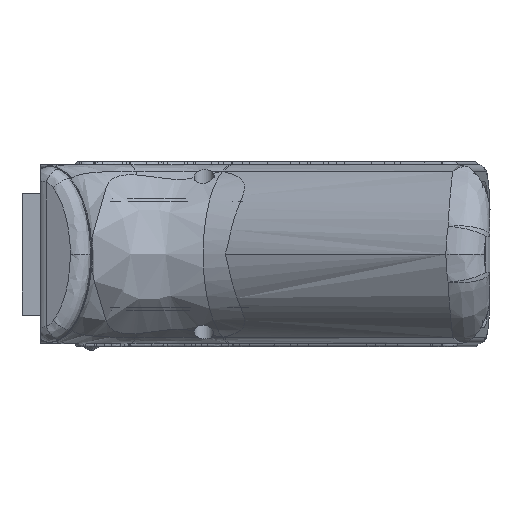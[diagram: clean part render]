
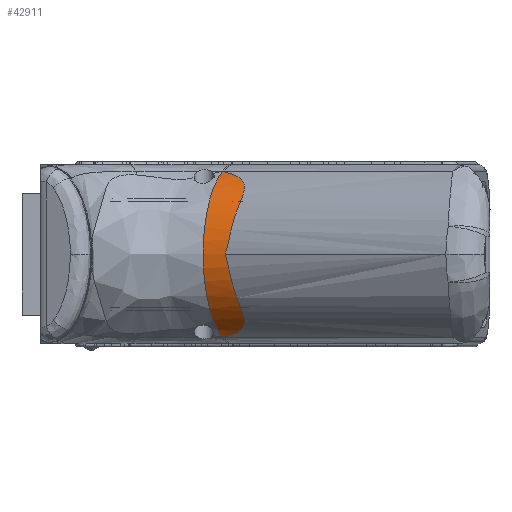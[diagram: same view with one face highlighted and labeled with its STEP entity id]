
A CAD part, left-side view. The second image highlights one B-rep face of the part: STEP entity #42911.
In plain terms, the highlighted free-form (B-spline) face has degree [2, 1] with [5, 2] control points.
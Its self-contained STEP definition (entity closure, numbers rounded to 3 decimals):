
#154=(
BOUNDED_SURFACE()
B_SPLINE_SURFACE(2,1,((#91286,#91287),(#91288,#91289),(#91290,#91291),(#91292,
#91293),(#91294,#91295)),.UNSPECIFIED.,.F.,.F.,.F.)
B_SPLINE_SURFACE_WITH_KNOTS((3,2,3),(2,2),(-2.705,-1.571,
-0.437),(0.,1.202),.UNSPECIFIED.)
GEOMETRIC_REPRESENTATION_ITEM()
RATIONAL_B_SPLINE_SURFACE(((1.,1.),(0.843,0.843),
(1.,1.),(0.843,0.843),(1.,1.)))
REPRESENTATION_ITEM('')
SURFACE()
);
#941=CIRCLE('',#45592,14.75);
#942=CIRCLE('',#45593,14.75);
#943=CIRCLE('',#45594,14.75);
#1328=B_SPLINE_CURVE_WITH_KNOTS('',3,(#60551,#60552,#60553,#60554,#60555,
#60556,#60557,#60558,#60559,#60560,#60561,#60562,#60563,#60564,#60565,#60566,
#60567,#60568,#60569,#60570,#60571,#60572,#60573,#60574,#60575,#60576,#60577,
#60578,#60579,#60580,#60581,#60582,#60583,#60584),.UNSPECIFIED.,.F.,.F.,
(4,2,2,2,2,2,2,2,2,2,2,2,2,2,2,2,4),(-1.682,-1.681,
-1.679,-1.676,-1.669,-1.656,
-1.628,-1.57,-1.446,-1.192,
-0.918,-0.77,-0.689,-0.595,
-0.408,-0.204,0.),.UNSPECIFIED.);
#1333=B_SPLINE_CURVE_WITH_KNOTS('',3,(#60663,#60664,#60665,#60666,#60667,
#60668,#60669,#60670,#60671,#60672,#60673,#60674,#60675,#60676,#60677,#60678,
#60679,#60680,#60681,#60682,#60683,#60684,#60685,#60686,#60687,#60688,#60689,
#60690,#60691,#60692,#60693,#60694,#60695,#60696),.UNSPECIFIED.,.F.,.F.,
(4,2,2,2,2,2,2,2,2,2,2,2,2,2,2,2,4),(-1.546,-1.327,
-1.203,-1.094,-1.026,-0.953,
-0.797,-0.662,-0.513,-0.26,
-0.125,-0.061,-0.03,-0.015,
-0.007,-0.004,0.),
 .UNSPECIFIED.);
#4348=FACE_OUTER_BOUND('',#7026,.T.);
#7026=EDGE_LOOP('',(#38418,#38419,#38420,#38421,#38422,#38423,#38424));
#11783=LINE('',#91296,#16512);
#11784=LINE('',#91297,#16513);
#16512=VECTOR('',#56331,10.);
#16513=VECTOR('',#56332,10.);
#17035=VERTEX_POINT('',#60548);
#17036=VERTEX_POINT('',#60550);
#17047=VERTEX_POINT('',#60661);
#20311=VERTEX_POINT('',#81430);
#20312=VERTEX_POINT('',#81432);
#20313=VERTEX_POINT('',#81434);
#20314=VERTEX_POINT('',#81436);
#21025=EDGE_CURVE('',#17035,#17036,#1328,.T.);
#21037=EDGE_CURVE('',#17047,#17035,#1333,.T.);
#26102=EDGE_CURVE('',#20312,#20311,#941,.T.);
#26103=EDGE_CURVE('',#20313,#20312,#942,.T.);
#26104=EDGE_CURVE('',#20314,#20313,#943,.T.);
#26525=EDGE_CURVE('',#20311,#17036,#11783,.T.);
#26526=EDGE_CURVE('',#20314,#17047,#11784,.T.);
#38418=ORIENTED_EDGE('',*,*,#26103,.T.);
#38419=ORIENTED_EDGE('',*,*,#26102,.T.);
#38420=ORIENTED_EDGE('',*,*,#26525,.T.);
#38421=ORIENTED_EDGE('',*,*,#21025,.F.);
#38422=ORIENTED_EDGE('',*,*,#21037,.F.);
#38423=ORIENTED_EDGE('',*,*,#26526,.F.);
#38424=ORIENTED_EDGE('',*,*,#26104,.T.);
#42911=ADVANCED_FACE('',(#4348),#154,.T.);
#45592=AXIS2_PLACEMENT_3D('',#81433,#55686,#55687);
#45593=AXIS2_PLACEMENT_3D('',#81435,#55688,#55689);
#45594=AXIS2_PLACEMENT_3D('',#81437,#55690,#55691);
#55686=DIRECTION('center_axis',(-0.367,-0.93,0.));
#55687=DIRECTION('ref_axis',(-0.393,0.155,0.906));
#55688=DIRECTION('center_axis',(-0.367,-0.93,0.));
#55689=DIRECTION('ref_axis',(-0.393,0.155,0.906));
#55690=DIRECTION('center_axis',(-0.367,-0.93,0.));
#55691=DIRECTION('ref_axis',(-0.393,0.155,0.906));
#56331=DIRECTION('',(-0.258,-0.966,0.));
#56332=DIRECTION('',(-0.258,-0.966,0.));
#60548=CARTESIAN_POINT('',(11.685,-31.202,0.));
#60550=CARTESIAN_POINT('',(20.555,-30.76,-13.366));
#60551=CARTESIAN_POINT('Ctrl Pts',(11.685,-31.202,0.));
#60552=CARTESIAN_POINT('Ctrl Pts',(11.684,-31.205,-0.01));
#60553=CARTESIAN_POINT('Ctrl Pts',(11.683,-31.208,-0.019));
#60554=CARTESIAN_POINT('Ctrl Pts',(11.682,-31.214,-0.038));
#60555=CARTESIAN_POINT('Ctrl Pts',(11.681,-31.217,-0.048));
#60556=CARTESIAN_POINT('Ctrl Pts',(11.679,-31.226,-0.077));
#60557=CARTESIAN_POINT('Ctrl Pts',(11.677,-31.231,-0.097));
#60558=CARTESIAN_POINT('Ctrl Pts',(11.673,-31.249,-0.155));
#60559=CARTESIAN_POINT('Ctrl Pts',(11.67,-31.261,-0.194));
#60560=CARTESIAN_POINT('Ctrl Pts',(11.663,-31.295,-0.313));
#60561=CARTESIAN_POINT('Ctrl Pts',(11.659,-31.318,-0.393));
#60562=CARTESIAN_POINT('Ctrl Pts',(11.649,-31.387,-0.637));
#60563=CARTESIAN_POINT('Ctrl Pts',(11.645,-31.431,-0.802));
#60564=CARTESIAN_POINT('Ctrl Pts',(11.644,-31.565,-1.316));
#60565=CARTESIAN_POINT('Ctrl Pts',(11.658,-31.648,-1.664));
#60566=CARTESIAN_POINT('Ctrl Pts',(11.745,-31.899,-2.752));
#60567=CARTESIAN_POINT('Ctrl Pts',(11.867,-32.053,-3.484));
#60568=CARTESIAN_POINT('Ctrl Pts',(12.396,-32.585,-5.68));
#60569=CARTESIAN_POINT('Ctrl Pts',(12.861,-32.988,-6.735));
#60570=CARTESIAN_POINT('Ctrl Pts',(13.504,-33.484,-8.043));
#60571=CARTESIAN_POINT('Ctrl Pts',(13.866,-33.728,-8.64));
#60572=CARTESIAN_POINT('Ctrl Pts',(14.445,-34.026,-9.448));
#60573=CARTESIAN_POINT('Ctrl Pts',(14.727,-34.156,-9.812));
#60574=CARTESIAN_POINT('Ctrl Pts',(15.241,-34.284,-10.371));
#60575=CARTESIAN_POINT('Ctrl Pts',(15.431,-34.312,-10.562));
#60576=CARTESIAN_POINT('Ctrl Pts',(15.862,-34.328,-10.96));
#60577=CARTESIAN_POINT('Ctrl Pts',(16.1,-34.308,-11.159));
#60578=CARTESIAN_POINT('Ctrl Pts',(16.839,-34.147,-11.721));
#60579=CARTESIAN_POINT('Ctrl Pts',(17.326,-33.914,-12.021));
#60580=CARTESIAN_POINT('Ctrl Pts',(18.319,-33.239,-12.548));
#60581=CARTESIAN_POINT('Ctrl Pts',(18.815,-32.784,-12.762));
#60582=CARTESIAN_POINT('Ctrl Pts',(19.719,-31.825,-13.107));
#60583=CARTESIAN_POINT('Ctrl Pts',(20.153,-31.294,-13.249));
#60584=CARTESIAN_POINT('Ctrl Pts',(20.555,-30.76,-13.366));
#60661=CARTESIAN_POINT('',(20.555,-30.76,13.366));
#60663=CARTESIAN_POINT('Ctrl Pts',(20.555,-30.76,13.366));
#60664=CARTESIAN_POINT('Ctrl Pts',(19.719,-31.872,13.121));
#60665=CARTESIAN_POINT('Ctrl Pts',(18.976,-32.662,12.842));
#60666=CARTESIAN_POINT('Ctrl Pts',(17.926,-33.522,12.346));
#60667=CARTESIAN_POINT('Ctrl Pts',(17.525,-33.792,12.134));
#60668=CARTESIAN_POINT('Ctrl Pts',(16.75,-34.155,11.648));
#60669=CARTESIAN_POINT('Ctrl Pts',(16.392,-34.26,11.393));
#60670=CARTESIAN_POINT('Ctrl Pts',(15.817,-34.321,10.918));
#60671=CARTESIAN_POINT('Ctrl Pts',(15.606,-34.318,10.727));
#60672=CARTESIAN_POINT('Ctrl Pts',(15.184,-34.267,10.311));
#60673=CARTESIAN_POINT('Ctrl Pts',(14.977,-34.216,10.088));
#60674=CARTESIAN_POINT('Ctrl Pts',(14.364,-34.009,9.363));
#60675=CARTESIAN_POINT('Ctrl Pts',(13.993,-33.796,8.832));
#60676=CARTESIAN_POINT('Ctrl Pts',(13.391,-33.396,7.817));
#60677=CARTESIAN_POINT('Ctrl Pts',(13.149,-33.204,7.339));
#60678=CARTESIAN_POINT('Ctrl Pts',(12.701,-32.829,6.323));
#60679=CARTESIAN_POINT('Ctrl Pts',(12.495,-32.645,5.771));
#60680=CARTESIAN_POINT('Ctrl Pts',(12.016,-32.203,4.231));
#60681=CARTESIAN_POINT('Ctrl Pts',(11.835,-32.014,3.329));
#60682=CARTESIAN_POINT('Ctrl Pts',(11.685,-31.74,2.075));
#60683=CARTESIAN_POINT('Ctrl Pts',(11.655,-31.642,1.638));
#60684=CARTESIAN_POINT('Ctrl Pts',(11.643,-31.481,0.994));
#60685=CARTESIAN_POINT('Ctrl Pts',(11.645,-31.428,0.788));
#60686=CARTESIAN_POINT('Ctrl Pts',(11.655,-31.344,0.484));
#60687=CARTESIAN_POINT('Ctrl Pts',(11.659,-31.316,0.386));
#60688=CARTESIAN_POINT('Ctrl Pts',(11.668,-31.274,0.239));
#60689=CARTESIAN_POINT('Ctrl Pts',(11.671,-31.26,0.191));
#60690=CARTESIAN_POINT('Ctrl Pts',(11.676,-31.238,0.119));
#60691=CARTESIAN_POINT('Ctrl Pts',(11.677,-31.231,0.095));
#60692=CARTESIAN_POINT('Ctrl Pts',(11.68,-31.22,0.059));
#60693=CARTESIAN_POINT('Ctrl Pts',(11.681,-31.217,0.047));
#60694=CARTESIAN_POINT('Ctrl Pts',(11.683,-31.209,0.024));
#60695=CARTESIAN_POINT('Ctrl Pts',(11.684,-31.206,0.012));
#60696=CARTESIAN_POINT('Ctrl Pts',(11.685,-31.202,0.));
#81430=CARTESIAN_POINT('',(20.555,-30.76,-13.366));
#81432=CARTESIAN_POINT('',(13.248,-27.881,-4.36));
#81433=CARTESIAN_POINT('Origin',(26.359,-33.046,0.));
#81434=CARTESIAN_POINT('',(13.248,-27.881,4.36));
#81435=CARTESIAN_POINT('Origin',(26.359,-33.046,0.));
#81436=CARTESIAN_POINT('',(20.555,-30.76,13.366));
#81437=CARTESIAN_POINT('Origin',(26.359,-33.046,0.));
#91286=CARTESIAN_POINT('Ctrl Pts',(20.812,-29.796,13.366));
#91287=CARTESIAN_POINT('Ctrl Pts',(17.714,-41.411,13.366));
#91288=CARTESIAN_POINT('Ctrl Pts',(12.641,-27.616,9.394));
#91289=CARTESIAN_POINT('Ctrl Pts',(9.543,-39.232,9.394));
#91290=CARTESIAN_POINT('Ctrl Pts',(12.641,-27.616,0.));
#91291=CARTESIAN_POINT('Ctrl Pts',(9.543,-39.232,0.));
#91292=CARTESIAN_POINT('Ctrl Pts',(12.641,-27.616,-9.394));
#91293=CARTESIAN_POINT('Ctrl Pts',(9.543,-39.232,-9.394));
#91294=CARTESIAN_POINT('Ctrl Pts',(20.812,-29.796,-13.366));
#91295=CARTESIAN_POINT('Ctrl Pts',(17.714,-41.411,-13.366));
#91296=CARTESIAN_POINT('',(20.555,-30.76,-13.366));
#91297=CARTESIAN_POINT('',(20.555,-30.76,13.366));
